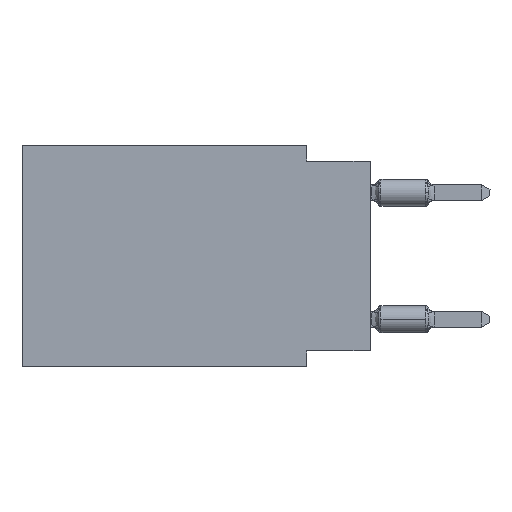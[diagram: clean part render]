
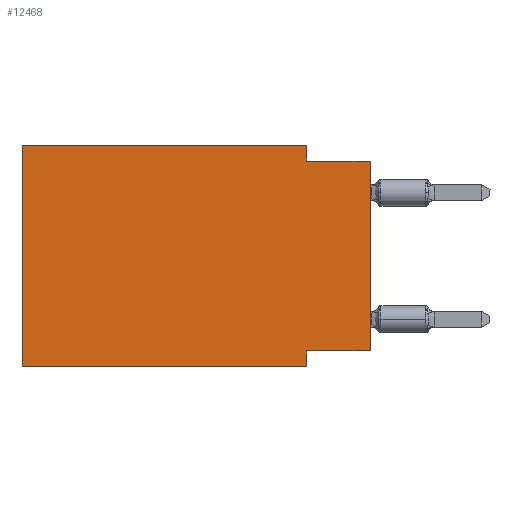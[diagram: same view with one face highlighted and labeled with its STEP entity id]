
A CAD part, left-side view. The second image highlights one B-rep face of the part: STEP entity #12468.
In plain terms, the highlighted planar face has unit normal (-1, 0, 0).
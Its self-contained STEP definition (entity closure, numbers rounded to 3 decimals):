
#2 = LINE ( 'NONE', #6286, #570 ) ;
#24 = LINE ( 'NONE', #16630, #2921 ) ;
#51 = EDGE_CURVE ( 'NONE', #4212, #8791, #16394, .T. ) ;
#570 = VECTOR ( 'NONE', #2550, 1000. ) ;
#916 = CARTESIAN_POINT ( 'NONE',  ( 0., 13.97, -8.89 ) ) ;
#1158 = DIRECTION ( 'NONE',  ( 0., 0., -1. ) ) ;
#1391 = EDGE_CURVE ( 'NONE', #12931, #5126, #3605, .T. ) ;
#1400 = CARTESIAN_POINT ( 'NONE',  ( 0., 2.54, -8.89 ) ) ;
#1502 = ORIENTED_EDGE ( 'NONE', *, *, #1733, .F. ) ;
#1733 = EDGE_CURVE ( 'NONE', #14807, #12234, #2, .T. ) ;
#1820 = CARTESIAN_POINT ( 'NONE',  ( 0., 0., -8.255 ) ) ;
#2263 = CARTESIAN_POINT ( 'NONE',  ( 0., 13.97, 0. ) ) ;
#2550 = DIRECTION ( 'NONE',  ( 0., 0., -1. ) ) ;
#2563 = VERTEX_POINT ( 'NONE', #2263 ) ;
#2921 = VECTOR ( 'NONE', #5028, 1000. ) ;
#3432 = DIRECTION ( 'NONE',  ( 0., -1., 0. ) ) ;
#3605 = LINE ( 'NONE', #8853, #4354 ) ;
#3982 = ORIENTED_EDGE ( 'NONE', *, *, #51, .T. ) ;
#4159 = PLANE ( 'NONE',  #11410 ) ;
#4212 = VERTEX_POINT ( 'NONE', #9935 ) ;
#4350 = CARTESIAN_POINT ( 'NONE',  ( 0., 2.54, -8.255 ) ) ;
#4354 = VECTOR ( 'NONE', #3432, 1000. ) ;
#4443 = CARTESIAN_POINT ( 'NONE',  ( 0., 2.54, 0. ) ) ;
#4458 = ORIENTED_EDGE ( 'NONE', *, *, #14700, .F. ) ;
#5028 = DIRECTION ( 'NONE',  ( 0., -1., 0. ) ) ;
#5126 = VERTEX_POINT ( 'NONE', #5509 ) ;
#5509 = CARTESIAN_POINT ( 'NONE',  ( 0., 2.54, -8.89 ) ) ;
#5657 = ORIENTED_EDGE ( 'NONE', *, *, #15304, .F. ) ;
#5970 = LINE ( 'NONE', #1820, #13908 ) ;
#6042 = VERTEX_POINT ( 'NONE', #4350 ) ;
#6286 = CARTESIAN_POINT ( 'NONE',  ( 0., 2.54, 0. ) ) ;
#7709 = CARTESIAN_POINT ( 'NONE',  ( 0., 0., -0.635 ) ) ;
#7794 = DIRECTION ( 'NONE',  ( 0., 0., 1. ) ) ;
#7899 = VECTOR ( 'NONE', #12593, 1000. ) ;
#8768 = EDGE_LOOP ( 'NONE', ( #3982, #5657, #1502, #9533, #11075, #12908, #4458, #12252 ) ) ;
#8791 = VERTEX_POINT ( 'NONE', #7709 ) ;
#8853 = CARTESIAN_POINT ( 'NONE',  ( 0., 13.97, -8.89 ) ) ;
#9155 = CARTESIAN_POINT ( 'NONE',  ( 0., 0., -0.635 ) ) ;
#9448 = CARTESIAN_POINT ( 'NONE',  ( 0., 2.54, -0.635 ) ) ;
#9533 = ORIENTED_EDGE ( 'NONE', *, *, #15108, .F. ) ;
#9935 = CARTESIAN_POINT ( 'NONE',  ( 0., 0., -8.255 ) ) ;
#9959 = CARTESIAN_POINT ( 'NONE',  ( 0., 0., 0. ) ) ;
#10782 = LINE ( 'NONE', #14688, #14037 ) ;
#10938 = CARTESIAN_POINT ( 'NONE',  ( 0., 13.97, 0. ) ) ;
#11013 = FACE_OUTER_BOUND ( 'NONE', #8768, .T. ) ;
#11075 = ORIENTED_EDGE ( 'NONE', *, *, #16029, .F. ) ;
#11121 = EDGE_CURVE ( 'NONE', #4212, #6042, #5970, .T. ) ;
#11410 = AXIS2_PLACEMENT_3D ( 'NONE', #10938, #14487, #14574 ) ;
#11569 = LINE ( 'NONE', #1400, #13201 ) ;
#12234 = VERTEX_POINT ( 'NONE', #9448 ) ;
#12252 = ORIENTED_EDGE ( 'NONE', *, *, #11121, .F. ) ;
#12468 = ADVANCED_FACE ( 'NONE', ( #11013 ), #4159, .F. ) ;
#12593 = DIRECTION ( 'NONE',  ( 0., 0., 1. ) ) ;
#12908 = ORIENTED_EDGE ( 'NONE', *, *, #1391, .T. ) ;
#12931 = VERTEX_POINT ( 'NONE', #916 ) ;
#13201 = VECTOR ( 'NONE', #1158, 1000. ) ;
#13908 = VECTOR ( 'NONE', #16210, 1000. ) ;
#14037 = VECTOR ( 'NONE', #7794, 1000. ) ;
#14487 = DIRECTION ( 'NONE',  ( 1., 0., 0. ) ) ;
#14490 = LINE ( 'NONE', #9155, #15631 ) ;
#14574 = DIRECTION ( 'NONE',  ( 0., 0., -1. ) ) ;
#14688 = CARTESIAN_POINT ( 'NONE',  ( 0., 13.97, 0. ) ) ;
#14700 = EDGE_CURVE ( 'NONE', #6042, #5126, #11569, .T. ) ;
#14807 = VERTEX_POINT ( 'NONE', #4443 ) ;
#15108 = EDGE_CURVE ( 'NONE', #2563, #14807, #24, .T. ) ;
#15304 = EDGE_CURVE ( 'NONE', #12234, #8791, #14490, .T. ) ;
#15631 = VECTOR ( 'NONE', #15837, 1000. ) ;
#15837 = DIRECTION ( 'NONE',  ( 0., -1., 0. ) ) ;
#16029 = EDGE_CURVE ( 'NONE', #12931, #2563, #10782, .T. ) ;
#16210 = DIRECTION ( 'NONE',  ( 0., 1., 0. ) ) ;
#16394 = LINE ( 'NONE', #9959, #7899 ) ;
#16630 = CARTESIAN_POINT ( 'NONE',  ( 0., 13.97, 0. ) ) ;
